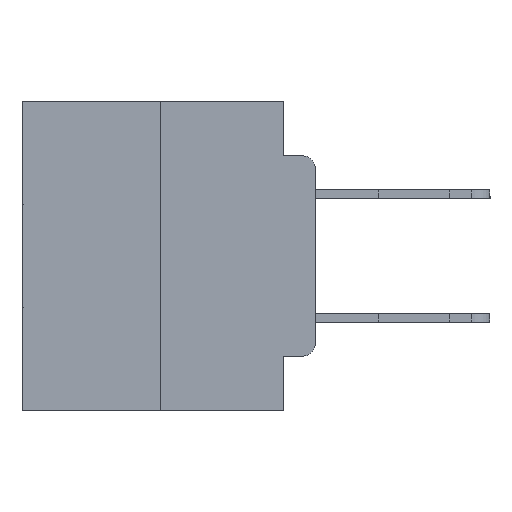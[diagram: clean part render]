
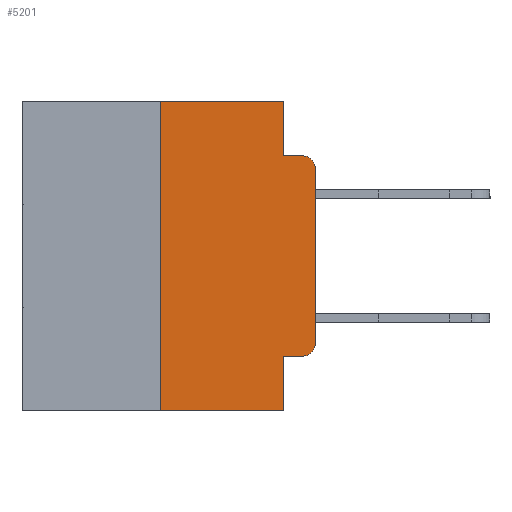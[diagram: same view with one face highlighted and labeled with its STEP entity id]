
A CAD part, left-side view. The second image highlights one B-rep face of the part: STEP entity #5201.
In plain terms, the highlighted planar face has unit normal (-1, 0, 0).
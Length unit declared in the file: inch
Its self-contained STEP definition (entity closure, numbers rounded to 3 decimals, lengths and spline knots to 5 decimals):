
#596 = AXIS2_PLACEMENT_3D ( 'NONE', #23289, #9856, #25520 ) ;
#785 = FACE_OUTER_BOUND ( 'NONE', #25385, .T. ) ;
#1159 = VERTEX_POINT ( 'NONE', #15727 ) ;
#1521 = CARTESIAN_POINT ( 'NONE',  ( 0., 0.25, 0. ) ) ;
#1764 = DIRECTION ( 'NONE',  ( 0., -1., 0. ) ) ;
#2556 = ORIENTED_EDGE ( 'NONE', *, *, #3602, .T. ) ;
#3452 = DIRECTION ( 'NONE',  ( 0., 0., -1. ) ) ;
#3454 = CARTESIAN_POINT ( 'NONE',  ( 0., 0.25, -0.5 ) ) ;
#3539 = DIRECTION ( 'NONE',  ( -1., 0., 0. ) ) ;
#3564 = CARTESIAN_POINT ( 'NONE',  ( 0., 0.02, -0.4115 ) ) ;
#3602 = EDGE_CURVE ( 'NONE', #12079, #21511, #12495, .T. ) ;
#3709 = LINE ( 'NONE', #28035, #20195 ) ;
#3730 = ORIENTED_EDGE ( 'NONE', *, *, #23716, .T. ) ;
#3991 = ORIENTED_EDGE ( 'NONE', *, *, #25212, .F. ) ;
#4226 = PLANE ( 'NONE',  #14706 ) ;
#4606 = VECTOR ( 'NONE', #22655, 39.37008 ) ;
#4778 = ORIENTED_EDGE ( 'NONE', *, *, #11688, .F. ) ;
#5201 = ADVANCED_FACE ( 'NONE', ( #785 ), #4226, .F. ) ;
#5489 = ORIENTED_EDGE ( 'NONE', *, *, #24938, .F. ) ;
#6227 = EDGE_CURVE ( 'NONE', #21998, #13223, #10580, .T. ) ;
#6353 = CARTESIAN_POINT ( 'NONE',  ( 0., 0.051, -0.0885 ) ) ;
#6354 = ORIENTED_EDGE ( 'NONE', *, *, #13203, .F. ) ;
#6468 = DIRECTION ( 'NONE',  ( 0., 0., -1. ) ) ;
#6471 = CARTESIAN_POINT ( 'NONE',  ( 0., 0., -0.1085 ) ) ;
#7058 = ORIENTED_EDGE ( 'NONE', *, *, #19954, .T. ) ;
#7203 = VERTEX_POINT ( 'NONE', #14890 ) ;
#7312 = ORIENTED_EDGE ( 'NONE', *, *, #7748, .F. ) ;
#7748 = EDGE_CURVE ( 'NONE', #21998, #8158, #26705, .T. ) ;
#8100 = CARTESIAN_POINT ( 'NONE',  ( 0., 0.473, -0.5 ) ) ;
#8158 = VERTEX_POINT ( 'NONE', #25288 ) ;
#8206 = AXIS2_PLACEMENT_3D ( 'NONE', #16990, #3539, #19248 ) ;
#8254 = CARTESIAN_POINT ( 'NONE',  ( 0., 0., -0.3915 ) ) ;
#8393 = ORIENTED_EDGE ( 'NONE', *, *, #6227, .T. ) ;
#8618 = ORIENTED_EDGE ( 'NONE', *, *, #10187, .T. ) ;
#9856 = DIRECTION ( 'NONE',  ( -1., 0., 0. ) ) ;
#10187 = EDGE_CURVE ( 'NONE', #13223, #12079, #27953, .T. ) ;
#10248 = DIRECTION ( 'NONE',  ( 0., 0., 1. ) ) ;
#10580 = LINE ( 'NONE', #27054, #4606 ) ;
#10652 = VECTOR ( 'NONE', #25978, 39.37008 ) ;
#11298 = CARTESIAN_POINT ( 'NONE',  ( 0., 0.051, 0. ) ) ;
#11688 = EDGE_CURVE ( 'NONE', #1159, #7203, #19252, .T. ) ;
#12079 = VERTEX_POINT ( 'NONE', #8254 ) ;
#12088 = VERTEX_POINT ( 'NONE', #12760 ) ;
#12250 = DIRECTION ( 'NONE',  ( 0., 0., 1. ) ) ;
#12495 = LINE ( 'NONE', #23416, #17761 ) ;
#12760 = CARTESIAN_POINT ( 'NONE',  ( 0., 0.02, -0.0885 ) ) ;
#13203 = EDGE_CURVE ( 'NONE', #27302, #18242, #3709, .T. ) ;
#13223 = VERTEX_POINT ( 'NONE', #3564 ) ;
#14181 = VECTOR ( 'NONE', #3452, 39.37008 ) ;
#14661 = CARTESIAN_POINT ( 'NONE',  ( 0., 0.051, 0. ) ) ;
#14706 = AXIS2_PLACEMENT_3D ( 'NONE', #26480, #19896, #6468 ) ;
#14890 = CARTESIAN_POINT ( 'NONE',  ( 0., 0.051, -0.0885 ) ) ;
#15727 = CARTESIAN_POINT ( 'NONE',  ( 0., 0.051, 0. ) ) ;
#16942 = CARTESIAN_POINT ( 'NONE',  ( 0., 0.051, -0.4115 ) ) ;
#16990 = CARTESIAN_POINT ( 'NONE',  ( 0., 0.02, -0.3915 ) ) ;
#17761 = VECTOR ( 'NONE', #12250, 39.37008 ) ;
#18242 = VERTEX_POINT ( 'NONE', #1521 ) ;
#18470 = VECTOR ( 'NONE', #25560, 39.37008 ) ;
#19159 = LINE ( 'NONE', #23330, #18470 ) ;
#19248 = DIRECTION ( 'NONE',  ( 0., 0., -1. ) ) ;
#19252 = LINE ( 'NONE', #11298, #24503 ) ;
#19896 = DIRECTION ( 'NONE',  ( 1., 0., 0. ) ) ;
#19954 = EDGE_CURVE ( 'NONE', #27302, #8158, #28377, .T. ) ;
#20195 = VECTOR ( 'NONE', #10248, 39.37008 ) ;
#21511 = VERTEX_POINT ( 'NONE', #6471 ) ;
#21998 = VERTEX_POINT ( 'NONE', #16942 ) ;
#22655 = DIRECTION ( 'NONE',  ( 0., -1., 0. ) ) ;
#23289 = CARTESIAN_POINT ( 'NONE',  ( 0., 0.02, -0.1085 ) ) ;
#23330 = CARTESIAN_POINT ( 'NONE',  ( 0., 0.473, 0. ) ) ;
#23342 = VECTOR ( 'NONE', #1764, 39.37008 ) ;
#23416 = CARTESIAN_POINT ( 'NONE',  ( 0., 0., 0. ) ) ;
#23716 = EDGE_CURVE ( 'NONE', #21511, #12088, #27513, .T. ) ;
#24063 = LINE ( 'NONE', #6353, #23342 ) ;
#24503 = VECTOR ( 'NONE', #24720, 39.37008 ) ;
#24720 = DIRECTION ( 'NONE',  ( 0., 0., -1. ) ) ;
#24938 = EDGE_CURVE ( 'NONE', #18242, #1159, #19159, .T. ) ;
#25212 = EDGE_CURVE ( 'NONE', #7203, #12088, #24063, .T. ) ;
#25288 = CARTESIAN_POINT ( 'NONE',  ( 0., 0.051, -0.5 ) ) ;
#25385 = EDGE_LOOP ( 'NONE', ( #2556, #3730, #3991, #4778, #5489, #6354, #7058, #7312, #8393, #8618 ) ) ;
#25520 = DIRECTION ( 'NONE',  ( 0., 0., -1. ) ) ;
#25560 = DIRECTION ( 'NONE',  ( 0., -1., 0. ) ) ;
#25978 = DIRECTION ( 'NONE',  ( 0., -1., 0. ) ) ;
#26480 = CARTESIAN_POINT ( 'NONE',  ( 0., 0.473, 0. ) ) ;
#26705 = LINE ( 'NONE', #14661, #14181 ) ;
#27054 = CARTESIAN_POINT ( 'NONE',  ( 0., 0.051, -0.4115 ) ) ;
#27302 = VERTEX_POINT ( 'NONE', #3454 ) ;
#27513 = CIRCLE ( 'NONE', #596, 0.02 ) ;
#27953 = CIRCLE ( 'NONE', #8206, 0.02 ) ;
#28035 = CARTESIAN_POINT ( 'NONE',  ( 0., 0.25, 0. ) ) ;
#28377 = LINE ( 'NONE', #8100, #10652 ) ;
